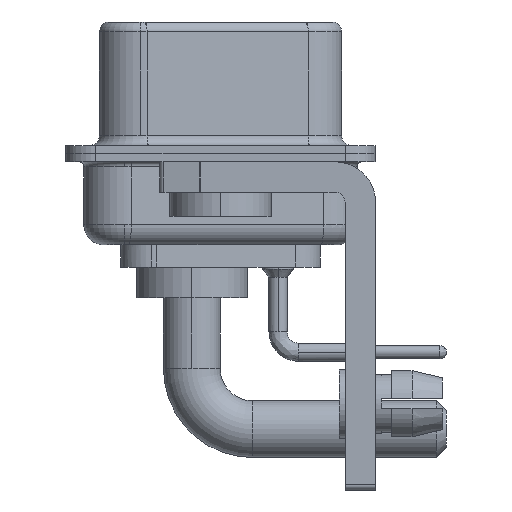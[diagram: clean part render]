
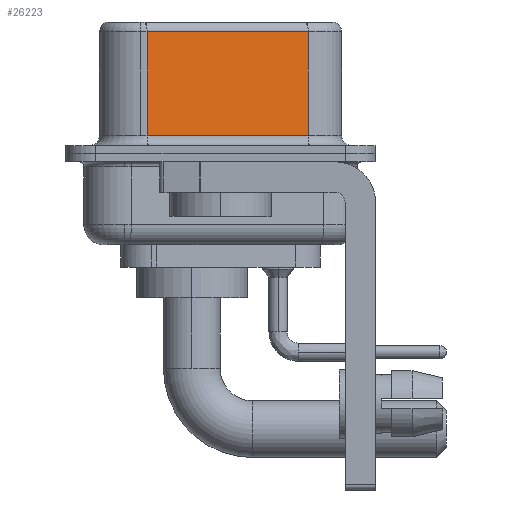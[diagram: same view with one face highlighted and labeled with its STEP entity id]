
A CAD part, left-side view. The second image highlights one B-rep face of the part: STEP entity #26223.
In plain terms, the highlighted planar face has unit normal (-0.985, -0.174, 0).
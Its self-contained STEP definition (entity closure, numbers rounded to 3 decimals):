
#954 = VECTOR ( 'NONE', #19409, 1000. ) ;
#1373 = DIRECTION ( 'NONE',  ( 0., 0., -1. ) ) ;
#1718 = VECTOR ( 'NONE', #20383, 1000. ) ;
#2096 = VECTOR ( 'NONE', #1373, 1000. ) ;
#2177 = CARTESIAN_POINT ( 'NONE',  ( 5.132, -4.322, 0.9 ) ) ;
#2378 = DIRECTION ( 'NONE',  ( 0.985, 0.174, 0. ) ) ;
#2985 = EDGE_CURVE ( 'NONE', #17318, #14258, #3114, .T. ) ;
#3098 = ORIENTED_EDGE ( 'NONE', *, *, #21852, .T. ) ;
#3114 = LINE ( 'NONE', #3505, #2096 ) ;
#3505 = CARTESIAN_POINT ( 'NONE',  ( 3.73, 3.628, 6.52 ) ) ;
#4633 = EDGE_CURVE ( 'NONE', #17116, #13502, #12061, .T. ) ;
#5438 = VECTOR ( 'NONE', #16627, 1000. ) ;
#6824 = CARTESIAN_POINT ( 'NONE',  ( 3.73, 3.628, 6.02 ) ) ;
#7645 = CARTESIAN_POINT ( 'NONE',  ( 3.73, 3.628, 0.9 ) ) ;
#9417 = AXIS2_PLACEMENT_3D ( 'NONE', #19102, #2378, #18710 ) ;
#10268 = ORIENTED_EDGE ( 'NONE', *, *, #2985, .T. ) ;
#11224 = CARTESIAN_POINT ( 'NONE',  ( 5.132, -4.322, 6.02 ) ) ;
#12061 = LINE ( 'NONE', #18509, #5438 ) ;
#13502 = VERTEX_POINT ( 'NONE', #14531 ) ;
#13621 = LINE ( 'NONE', #11224, #954 ) ;
#14229 = ORIENTED_EDGE ( 'NONE', *, *, #4633, .F. ) ;
#14258 = VERTEX_POINT ( 'NONE', #7645 ) ;
#14531 = CARTESIAN_POINT ( 'NONE',  ( 5.132, -4.322, 0.9 ) ) ;
#14555 = FACE_OUTER_BOUND ( 'NONE', #15805, .T. ) ;
#14942 = PLANE ( 'NONE',  #9417 ) ;
#15805 = EDGE_LOOP ( 'NONE', ( #14229, #3098, #10268, #20656 ) ) ;
#16358 = LINE ( 'NONE', #2177, #1718 ) ;
#16627 = DIRECTION ( 'NONE',  ( 0., 0., -1. ) ) ;
#17116 = VERTEX_POINT ( 'NONE', #20905 ) ;
#17318 = VERTEX_POINT ( 'NONE', #6824 ) ;
#18509 = CARTESIAN_POINT ( 'NONE',  ( 5.132, -4.322, 6.52 ) ) ;
#18710 = DIRECTION ( 'NONE',  ( -0.174, 0.985, 0. ) ) ;
#19102 = CARTESIAN_POINT ( 'NONE',  ( 5.132, -4.322, 6.52 ) ) ;
#19296 = EDGE_CURVE ( 'NONE', #14258, #13502, #16358, .T. ) ;
#19409 = DIRECTION ( 'NONE',  ( -0.174, 0.985, 0. ) ) ;
#20383 = DIRECTION ( 'NONE',  ( 0.174, -0.985, 0. ) ) ;
#20656 = ORIENTED_EDGE ( 'NONE', *, *, #19296, .T. ) ;
#20905 = CARTESIAN_POINT ( 'NONE',  ( 5.132, -4.322, 6.02 ) ) ;
#21852 = EDGE_CURVE ( 'NONE', #17116, #17318, #13621, .T. ) ;
#26223 = ADVANCED_FACE ( 'NONE', ( #14555 ), #14942, .F. ) ;
